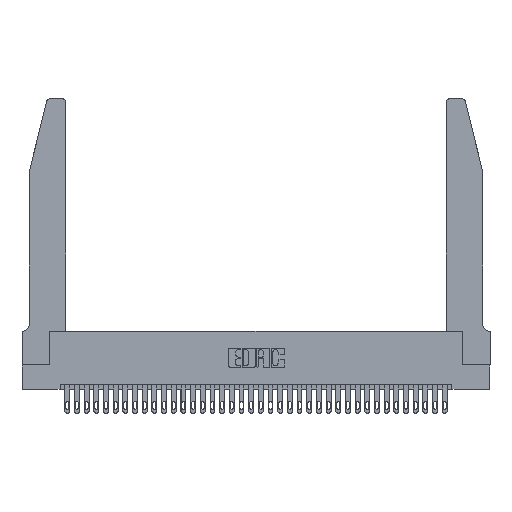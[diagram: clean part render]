
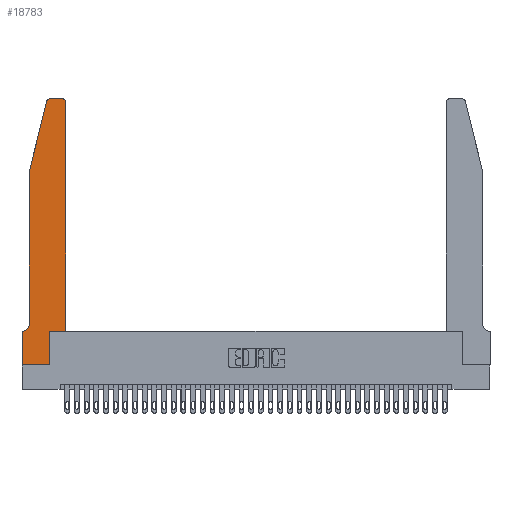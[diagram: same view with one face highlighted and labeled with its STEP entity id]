
A CAD part, top view. The second image highlights one B-rep face of the part: STEP entity #18783.
In plain terms, the highlighted planar face has unit normal (0, 0, 1).
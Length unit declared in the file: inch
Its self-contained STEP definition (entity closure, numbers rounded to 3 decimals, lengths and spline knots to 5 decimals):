
#211 = EDGE_CURVE ( 'NONE', #23818, #36157, #6736, .T. ) ;
#277 = EDGE_CURVE ( 'NONE', #21052, #2004, #35743, .T. ) ;
#519 = DIRECTION ( 'NONE',  ( 0., -1., 0. ) ) ;
#1582 = EDGE_CURVE ( 'NONE', #17433, #28128, #23311, .T. ) ;
#1646 = CARTESIAN_POINT ( 'NONE',  ( 0.284, 2.72, 0.37 ) ) ;
#2004 = VERTEX_POINT ( 'NONE', #23607 ) ;
#2471 = CARTESIAN_POINT ( 'NONE',  ( 0.4205, 2.75, 0.37 ) ) ;
#3189 = CARTESIAN_POINT ( 'NONE',  ( 0., 0., 0.37 ) ) ;
#3915 = CIRCLE ( 'NONE', #6978, 0.07 ) ;
#4674 = PLANE ( 'NONE',  #23578 ) ;
#6442 = CARTESIAN_POINT ( 'NONE',  ( 0.4505, 2.72, 0.37 ) ) ;
#6736 = CIRCLE ( 'NONE', #21034, 0.03 ) ;
#6916 = CARTESIAN_POINT ( 'NONE',  ( 0.4505, 0.35, 0.37 ) ) ;
#6978 = AXIS2_PLACEMENT_3D ( 'NONE', #29515, #13108, #24132 ) ;
#7109 = DIRECTION ( 'NONE',  ( 0., 0., 1. ) ) ;
#7353 = CARTESIAN_POINT ( 'NONE',  ( 0.284, 2.75, 0.37 ) ) ;
#7993 = DIRECTION ( 'NONE',  ( -1., 0., 0. ) ) ;
#8382 = EDGE_CURVE ( 'NONE', #2004, #23818, #29614, .T. ) ;
#8876 = ORIENTED_EDGE ( 'NONE', *, *, #1582, .T. ) ;
#10133 = VECTOR ( 'NONE', #36033, 39.37008 ) ;
#11008 = EDGE_CURVE ( 'NONE', #17976, #21355, #17568, .T. ) ;
#12111 = DIRECTION ( 'NONE',  ( 0., 0., 1. ) ) ;
#12112 = VERTEX_POINT ( 'NONE', #17420 ) ;
#12604 = CARTESIAN_POINT ( 'NONE',  ( 0., 0.35, 0.37 ) ) ;
#12903 = ORIENTED_EDGE ( 'NONE', *, *, #35811, .T. ) ;
#13003 = ORIENTED_EDGE ( 'NONE', *, *, #34008, .T. ) ;
#13108 = DIRECTION ( 'NONE',  ( 0., 0., -1. ) ) ;
#13415 = ORIENTED_EDGE ( 'NONE', *, *, #277, .T. ) ;
#13527 = DIRECTION ( 'NONE',  ( 1., 0., 0. ) ) ;
#13650 = DIRECTION ( 'NONE',  ( -0.239, -0.971, 0. ) ) ;
#14425 = EDGE_CURVE ( 'NONE', #20891, #21052, #20355, .T. ) ;
#15065 = CARTESIAN_POINT ( 'NONE',  ( 0.4205, 2.72, 0.37 ) ) ;
#15280 = VECTOR ( 'NONE', #13650, 39.37008 ) ;
#15593 = CARTESIAN_POINT ( 'NONE',  ( 0.2865, 0., 0.37 ) ) ;
#16592 = CARTESIAN_POINT ( 'NONE',  ( 0.0755, 2., 0.37 ) ) ;
#16658 = CIRCLE ( 'NONE', #22320, 0.03 ) ;
#17161 = EDGE_CURVE ( 'NONE', #12112, #20891, #33826, .T. ) ;
#17220 = ORIENTED_EDGE ( 'NONE', *, *, #17161, .T. ) ;
#17310 = ORIENTED_EDGE ( 'NONE', *, *, #211, .T. ) ;
#17333 = EDGE_LOOP ( 'NONE', ( #12903, #27345, #23821, #18341, #13003, #8876, #26897, #17220, #35067, #13415, #36322, #17310 ) ) ;
#17420 = CARTESIAN_POINT ( 'NONE',  ( 0., 0., 0.37 ) ) ;
#17433 = VERTEX_POINT ( 'NONE', #19309 ) ;
#17568 = LINE ( 'NONE', #22286, #10133 ) ;
#17875 = CARTESIAN_POINT ( 'NONE',  ( 0.0755, 0.42, 0.37 ) ) ;
#17976 = VERTEX_POINT ( 'NONE', #16592 ) ;
#18341 = ORIENTED_EDGE ( 'NONE', *, *, #11008, .T. ) ;
#18384 = DIRECTION ( 'NONE',  ( 0., 1., 0. ) ) ;
#18715 = LINE ( 'NONE', #3189, #35825 ) ;
#18783 = ADVANCED_FACE ( 'NONE', ( #26157 ), #4674, .T. ) ;
#19100 = CARTESIAN_POINT ( 'NONE',  ( 0., 0., 0.37 ) ) ;
#19309 = CARTESIAN_POINT ( 'NONE',  ( 0.0055, 0.35, 0.37 ) ) ;
#19659 = CARTESIAN_POINT ( 'NONE',  ( 0.25487, 2.72718, 0.37 ) ) ;
#20355 = LINE ( 'NONE', #32328, #31690 ) ;
#20583 = CARTESIAN_POINT ( 'NONE',  ( 0.2605, 2.75, 0.37 ) ) ;
#20891 = VERTEX_POINT ( 'NONE', #15593 ) ;
#21034 = AXIS2_PLACEMENT_3D ( 'NONE', #15065, #12111, #31575 ) ;
#21052 = VERTEX_POINT ( 'NONE', #36098 ) ;
#21355 = VERTEX_POINT ( 'NONE', #17875 ) ;
#21477 = EDGE_CURVE ( 'NONE', #34697, #36211, #16658, .T. ) ;
#21489 = CARTESIAN_POINT ( 'NONE',  ( 0.4505, 0.35, 0.37 ) ) ;
#22286 = CARTESIAN_POINT ( 'NONE',  ( 0.0755, 2., 0.37 ) ) ;
#22320 = AXIS2_PLACEMENT_3D ( 'NONE', #1646, #7109, #35023 ) ;
#22704 = VECTOR ( 'NONE', #23401, 39.37008 ) ;
#23241 = VECTOR ( 'NONE', #35356, 39.37008 ) ;
#23273 = EDGE_CURVE ( 'NONE', #28128, #12112, #18715, .T. ) ;
#23311 = LINE ( 'NONE', #24761, #25492 ) ;
#23401 = DIRECTION ( 'NONE',  ( -1., 0., 0. ) ) ;
#23578 = AXIS2_PLACEMENT_3D ( 'NONE', #27435, #30157, #29903 ) ;
#23607 = CARTESIAN_POINT ( 'NONE',  ( 0.4505, 0.35, 0.37 ) ) ;
#23818 = VERTEX_POINT ( 'NONE', #6442 ) ;
#23821 = ORIENTED_EDGE ( 'NONE', *, *, #28185, .T. ) ;
#24132 = DIRECTION ( 'NONE',  ( -1., 0., 0. ) ) ;
#24761 = CARTESIAN_POINT ( 'NONE',  ( 0.0755, 0.35, 0.37 ) ) ;
#25492 = VECTOR ( 'NONE', #7993, 39.37008 ) ;
#26157 = FACE_OUTER_BOUND ( 'NONE', #17333, .T. ) ;
#26486 = DIRECTION ( 'NONE',  ( 0., 1., 0. ) ) ;
#26897 = ORIENTED_EDGE ( 'NONE', *, *, #23273, .T. ) ;
#26927 = VECTOR ( 'NONE', #13527, 39.37008 ) ;
#27345 = ORIENTED_EDGE ( 'NONE', *, *, #21477, .T. ) ;
#27435 = CARTESIAN_POINT ( 'NONE',  ( 0., 0.35, 0.37 ) ) ;
#28128 = VERTEX_POINT ( 'NONE', #12604 ) ;
#28185 = EDGE_CURVE ( 'NONE', #36211, #17976, #30231, .T. ) ;
#29515 = CARTESIAN_POINT ( 'NONE',  ( 0.0055, 0.42, 0.37 ) ) ;
#29614 = LINE ( 'NONE', #6916, #30053 ) ;
#29903 = DIRECTION ( 'NONE',  ( 1., 0., 0. ) ) ;
#30053 = VECTOR ( 'NONE', #26486, 39.37008 ) ;
#30157 = DIRECTION ( 'NONE',  ( 0., 0., 1. ) ) ;
#30184 = CARTESIAN_POINT ( 'NONE',  ( 0.0755, 2., 0.37 ) ) ;
#30231 = LINE ( 'NONE', #30184, #15280 ) ;
#31575 = DIRECTION ( 'NONE',  ( 1., 0., 0. ) ) ;
#31690 = VECTOR ( 'NONE', #18384, 39.37008 ) ;
#32328 = CARTESIAN_POINT ( 'NONE',  ( 0.2865, 0.35, 0.37 ) ) ;
#33668 = LINE ( 'NONE', #20583, #22704 ) ;
#33826 = LINE ( 'NONE', #19100, #23241 ) ;
#34008 = EDGE_CURVE ( 'NONE', #21355, #17433, #3915, .T. ) ;
#34697 = VERTEX_POINT ( 'NONE', #7353 ) ;
#35023 = DIRECTION ( 'NONE',  ( 1., 0., 0. ) ) ;
#35067 = ORIENTED_EDGE ( 'NONE', *, *, #14425, .T. ) ;
#35356 = DIRECTION ( 'NONE',  ( 1., 0., 0. ) ) ;
#35743 = LINE ( 'NONE', #21489, #26927 ) ;
#35811 = EDGE_CURVE ( 'NONE', #36157, #34697, #33668, .T. ) ;
#35825 = VECTOR ( 'NONE', #519, 39.37008 ) ;
#36033 = DIRECTION ( 'NONE',  ( 0., -1., 0. ) ) ;
#36098 = CARTESIAN_POINT ( 'NONE',  ( 0.2865, 0.35, 0.37 ) ) ;
#36157 = VERTEX_POINT ( 'NONE', #2471 ) ;
#36211 = VERTEX_POINT ( 'NONE', #19659 ) ;
#36322 = ORIENTED_EDGE ( 'NONE', *, *, #8382, .T. ) ;
